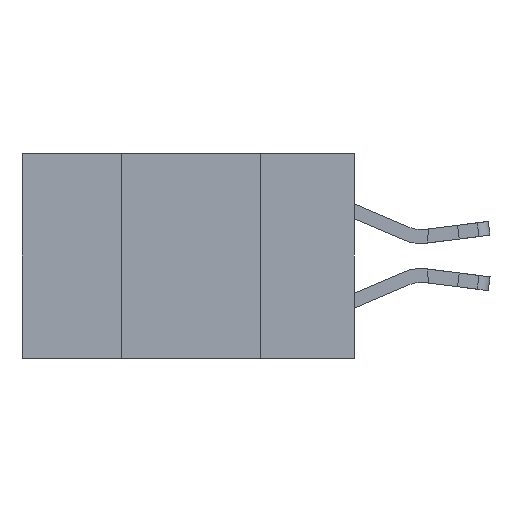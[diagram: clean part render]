
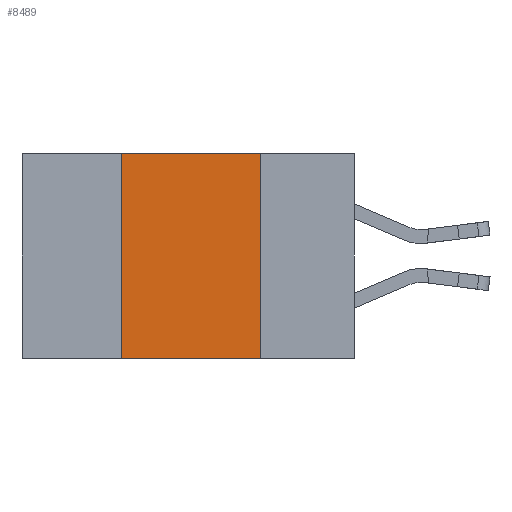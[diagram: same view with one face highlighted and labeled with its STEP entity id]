
A CAD part, left-side view. The second image highlights one B-rep face of the part: STEP entity #8489.
In plain terms, the highlighted planar face has unit normal (-1, 0, 0).
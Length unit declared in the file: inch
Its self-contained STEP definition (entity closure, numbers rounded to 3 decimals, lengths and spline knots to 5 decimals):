
#321 = CARTESIAN_POINT ( 'NONE',  ( 0., 0.17, 0. ) ) ;
#350 = ORIENTED_EDGE ( 'NONE', *, *, #16886, .F. ) ;
#905 = CARTESIAN_POINT ( 'NONE',  ( 0., 0.6, -0.37 ) ) ;
#929 = CARTESIAN_POINT ( 'NONE',  ( 0., 0.42, 0. ) ) ;
#1126 = VERTEX_POINT ( 'NONE', #929 ) ;
#2793 = LINE ( 'NONE', #11098, #6017 ) ;
#3758 = DIRECTION ( 'NONE',  ( 0., 0., -1. ) ) ;
#3819 = PLANE ( 'NONE',  #5679 ) ;
#4430 = ORIENTED_EDGE ( 'NONE', *, *, #7070, .F. ) ;
#4512 = CARTESIAN_POINT ( 'NONE',  ( 0., 0.6, 0. ) ) ;
#4541 = VECTOR ( 'NONE', #8013, 39.37008 ) ;
#5053 = VECTOR ( 'NONE', #17006, 39.37008 ) ;
#5596 = ORIENTED_EDGE ( 'NONE', *, *, #10508, .F. ) ;
#5679 = AXIS2_PLACEMENT_3D ( 'NONE', #4512, #7059, #3758 ) ;
#5845 = VECTOR ( 'NONE', #9646, 39.37008 ) ;
#6017 = VECTOR ( 'NONE', #11572, 39.37008 ) ;
#6084 = EDGE_LOOP ( 'NONE', ( #5596, #4430, #350, #15361 ) ) ;
#6566 = VERTEX_POINT ( 'NONE', #17104 ) ;
#7059 = DIRECTION ( 'NONE',  ( 1., 0., 0. ) ) ;
#7070 = EDGE_CURVE ( 'NONE', #1126, #17173, #16053, .T. ) ;
#8013 = DIRECTION ( 'NONE',  ( 0., 0., 1. ) ) ;
#8489 = ADVANCED_FACE ( 'NONE', ( #15213 ), #3819, .F. ) ;
#8609 = LINE ( 'NONE', #14636, #4541 ) ;
#9409 = CARTESIAN_POINT ( 'NONE',  ( 0., 0.17, -0.37 ) ) ;
#9608 = CARTESIAN_POINT ( 'NONE',  ( 0., 0.6, 0. ) ) ;
#9646 = DIRECTION ( 'NONE',  ( 0., -1., 0. ) ) ;
#10508 = EDGE_CURVE ( 'NONE', #17173, #12293, #2793, .T. ) ;
#11098 = CARTESIAN_POINT ( 'NONE',  ( 0., 0.17, -0.37 ) ) ;
#11572 = DIRECTION ( 'NONE',  ( 0., 0., -1. ) ) ;
#12293 = VERTEX_POINT ( 'NONE', #9409 ) ;
#12320 = LINE ( 'NONE', #905, #5053 ) ;
#12830 = EDGE_CURVE ( 'NONE', #6566, #12293, #12320, .T. ) ;
#14636 = CARTESIAN_POINT ( 'NONE',  ( 0., 0.42, -0.37 ) ) ;
#15213 = FACE_OUTER_BOUND ( 'NONE', #6084, .T. ) ;
#15361 = ORIENTED_EDGE ( 'NONE', *, *, #12830, .T. ) ;
#16053 = LINE ( 'NONE', #9608, #5845 ) ;
#16886 = EDGE_CURVE ( 'NONE', #6566, #1126, #8609, .T. ) ;
#17006 = DIRECTION ( 'NONE',  ( 0., -1., 0. ) ) ;
#17104 = CARTESIAN_POINT ( 'NONE',  ( 0., 0.42, -0.37 ) ) ;
#17173 = VERTEX_POINT ( 'NONE', #321 ) ;
